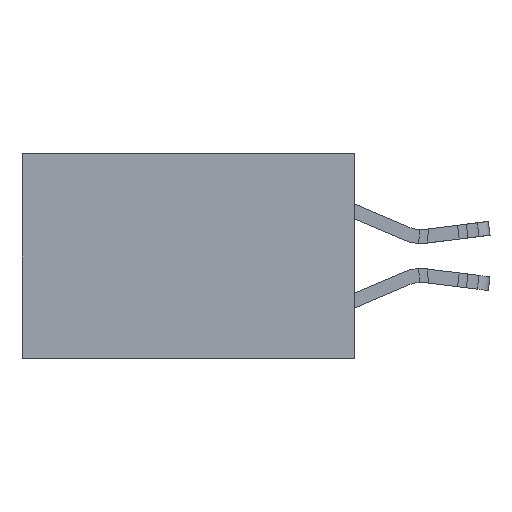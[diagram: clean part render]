
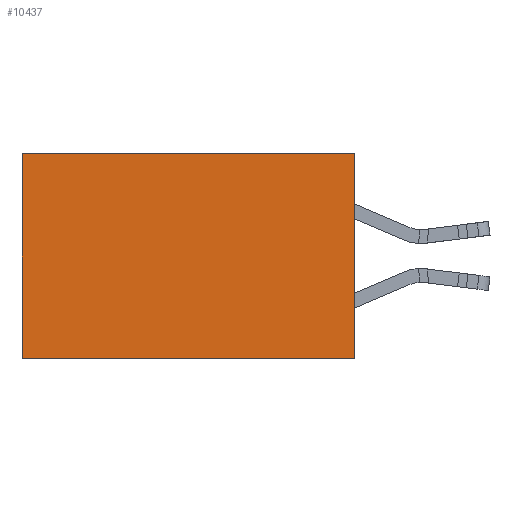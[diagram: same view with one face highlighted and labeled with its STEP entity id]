
A CAD part, left-side view. The second image highlights one B-rep face of the part: STEP entity #10437.
In plain terms, the highlighted planar face has unit normal (-1, 0, 0).
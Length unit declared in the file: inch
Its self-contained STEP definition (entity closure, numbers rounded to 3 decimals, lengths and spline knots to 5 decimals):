
#508 = DIRECTION ( 'NONE',  ( 0., 0., -1. ) ) ;
#2477 = ORIENTED_EDGE ( 'NONE', *, *, #8487, .F. ) ;
#2747 = ORIENTED_EDGE ( 'NONE', *, *, #15640, .T. ) ;
#4061 = CARTESIAN_POINT ( 'NONE',  ( 0.2615, 0., -0.37 ) ) ;
#4072 = CARTESIAN_POINT ( 'NONE',  ( 0.2615, 0., 0. ) ) ;
#5015 = CARTESIAN_POINT ( 'NONE',  ( 0.2615, 0.6, -0.37 ) ) ;
#6125 = LINE ( 'NONE', #4061, #13874 ) ;
#6488 = VERTEX_POINT ( 'NONE', #24340 ) ;
#7081 = VECTOR ( 'NONE', #508, 39.37008 ) ;
#7329 = DIRECTION ( 'NONE',  ( 0., 0., -1. ) ) ;
#7622 = CARTESIAN_POINT ( 'NONE',  ( 0.2615, 0., 0. ) ) ;
#7897 = EDGE_CURVE ( 'NONE', #26622, #16595, #13669, .T. ) ;
#8487 = EDGE_CURVE ( 'NONE', #26622, #6488, #10918, .T. ) ;
#10437 = ADVANCED_FACE ( 'NONE', ( #19942 ), #11833, .F. ) ;
#10918 = LINE ( 'NONE', #19291, #7081 ) ;
#11833 = PLANE ( 'NONE',  #14485 ) ;
#12670 = EDGE_CURVE ( 'NONE', #6488, #20727, #6125, .T. ) ;
#13669 = LINE ( 'NONE', #7622, #21871 ) ;
#13757 = DIRECTION ( 'NONE',  ( 0., 0., -1. ) ) ;
#13874 = VECTOR ( 'NONE', #20939, 39.37008 ) ;
#14485 = AXIS2_PLACEMENT_3D ( 'NONE', #17901, #22271, #13757 ) ;
#15640 = EDGE_CURVE ( 'NONE', #16595, #20727, #19818, .T. ) ;
#15982 = ORIENTED_EDGE ( 'NONE', *, *, #12670, .F. ) ;
#16595 = VERTEX_POINT ( 'NONE', #24783 ) ;
#17901 = CARTESIAN_POINT ( 'NONE',  ( 0.2615, 0., -0.37 ) ) ;
#18279 = VECTOR ( 'NONE', #7329, 39.37008 ) ;
#19291 = CARTESIAN_POINT ( 'NONE',  ( 0.2615, 0., -0.37 ) ) ;
#19818 = LINE ( 'NONE', #26144, #18279 ) ;
#19853 = DIRECTION ( 'NONE',  ( 0., 1., 0. ) ) ;
#19942 = FACE_OUTER_BOUND ( 'NONE', #25976, .T. ) ;
#20727 = VERTEX_POINT ( 'NONE', #5015 ) ;
#20939 = DIRECTION ( 'NONE',  ( 0., 1., 0. ) ) ;
#21871 = VECTOR ( 'NONE', #19853, 39.37008 ) ;
#22271 = DIRECTION ( 'NONE',  ( 1., 0., 0. ) ) ;
#24340 = CARTESIAN_POINT ( 'NONE',  ( 0.2615, 0., -0.37 ) ) ;
#24567 = ORIENTED_EDGE ( 'NONE', *, *, #7897, .T. ) ;
#24783 = CARTESIAN_POINT ( 'NONE',  ( 0.2615, 0.6, 0. ) ) ;
#25976 = EDGE_LOOP ( 'NONE', ( #2747, #15982, #2477, #24567 ) ) ;
#26144 = CARTESIAN_POINT ( 'NONE',  ( 0.2615, 0.6, -0.37 ) ) ;
#26622 = VERTEX_POINT ( 'NONE', #4072 ) ;
